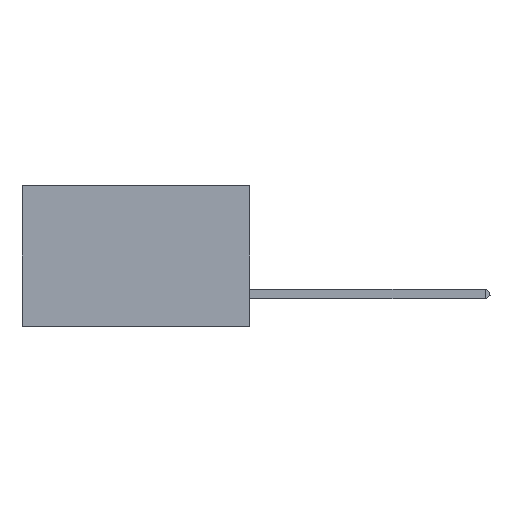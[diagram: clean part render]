
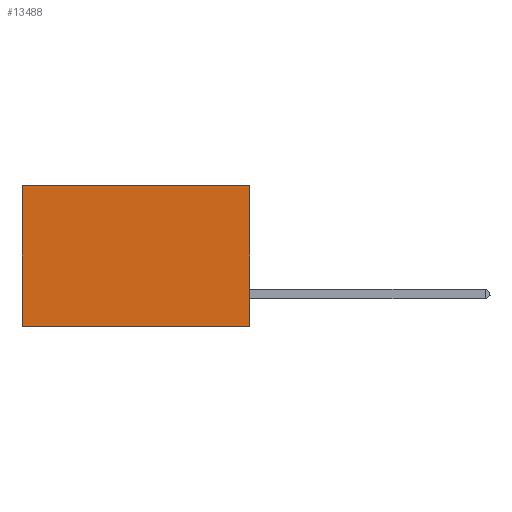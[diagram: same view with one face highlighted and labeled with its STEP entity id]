
A CAD part, left-side view. The second image highlights one B-rep face of the part: STEP entity #13488.
In plain terms, the highlighted planar face has unit normal (-1, 0, 0).
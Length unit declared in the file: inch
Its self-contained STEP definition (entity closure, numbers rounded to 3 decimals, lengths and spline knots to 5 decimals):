
#133 = LINE ( 'NONE', #11647, #10793 ) ;
#170 = VERTEX_POINT ( 'NONE', #2529 ) ;
#471 = ORIENTED_EDGE ( 'NONE', *, *, #9812, .T. ) ;
#1143 = VECTOR ( 'NONE', #5106, 39.37008 ) ;
#2386 = PLANE ( 'NONE',  #9134 ) ;
#2529 = CARTESIAN_POINT ( 'NONE',  ( 0.2875, 0.6, -0.37 ) ) ;
#2605 = VERTEX_POINT ( 'NONE', #10876 ) ;
#2648 = FACE_OUTER_BOUND ( 'NONE', #6531, .T. ) ;
#3043 = EDGE_CURVE ( 'NONE', #7565, #170, #133, .T. ) ;
#3508 = CARTESIAN_POINT ( 'NONE',  ( 0.2875, 0., 0. ) ) ;
#3945 = CARTESIAN_POINT ( 'NONE',  ( 0.2875, 0.6, 0. ) ) ;
#4183 = ORIENTED_EDGE ( 'NONE', *, *, #3043, .T. ) ;
#4407 = DIRECTION ( 'NONE',  ( 1., 0., 0. ) ) ;
#4750 = VERTEX_POINT ( 'NONE', #7238 ) ;
#5106 = DIRECTION ( 'NONE',  ( 0., 0., -1. ) ) ;
#5212 = CARTESIAN_POINT ( 'NONE',  ( 0.2875, 0., 0. ) ) ;
#6531 = EDGE_LOOP ( 'NONE', ( #4183, #9002, #8413, #471 ) ) ;
#7009 = VECTOR ( 'NONE', #8959, 39.37008 ) ;
#7238 = CARTESIAN_POINT ( 'NONE',  ( 0.2875, 0., 0. ) ) ;
#7286 = DIRECTION ( 'NONE',  ( 0., 0., -1. ) ) ;
#7565 = VERTEX_POINT ( 'NONE', #3945 ) ;
#8001 = LINE ( 'NONE', #3508, #7009 ) ;
#8290 = EDGE_CURVE ( 'NONE', #2605, #170, #10761, .T. ) ;
#8413 = ORIENTED_EDGE ( 'NONE', *, *, #12636, .F. ) ;
#8959 = DIRECTION ( 'NONE',  ( 0., 1., 0. ) ) ;
#9002 = ORIENTED_EDGE ( 'NONE', *, *, #8290, .F. ) ;
#9134 = AXIS2_PLACEMENT_3D ( 'NONE', #12167, #4407, #13110 ) ;
#9812 = EDGE_CURVE ( 'NONE', #4750, #7565, #8001, .T. ) ;
#10380 = VECTOR ( 'NONE', #12593, 39.37008 ) ;
#10420 = LINE ( 'NONE', #5212, #1143 ) ;
#10518 = CARTESIAN_POINT ( 'NONE',  ( 0.2875, 0., -0.37 ) ) ;
#10761 = LINE ( 'NONE', #10518, #10380 ) ;
#10793 = VECTOR ( 'NONE', #7286, 39.37008 ) ;
#10876 = CARTESIAN_POINT ( 'NONE',  ( 0.2875, 0., -0.37 ) ) ;
#11647 = CARTESIAN_POINT ( 'NONE',  ( 0.2875, 0.6, 0. ) ) ;
#12167 = CARTESIAN_POINT ( 'NONE',  ( 0.2875, 0., 0. ) ) ;
#12593 = DIRECTION ( 'NONE',  ( 0., 1., 0. ) ) ;
#12636 = EDGE_CURVE ( 'NONE', #4750, #2605, #10420, .T. ) ;
#13110 = DIRECTION ( 'NONE',  ( 0., 0., -1. ) ) ;
#13488 = ADVANCED_FACE ( 'NONE', ( #2648 ), #2386, .F. ) ;
